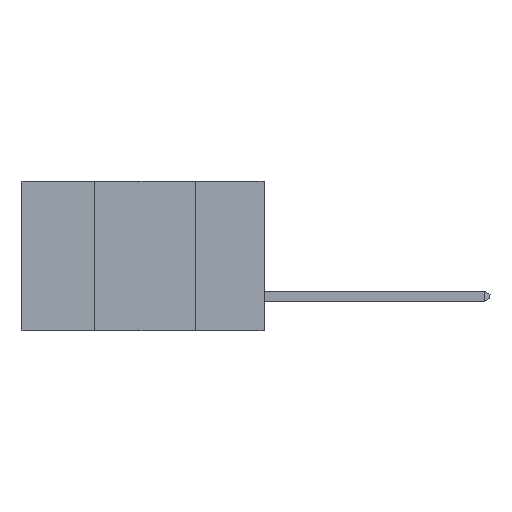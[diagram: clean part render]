
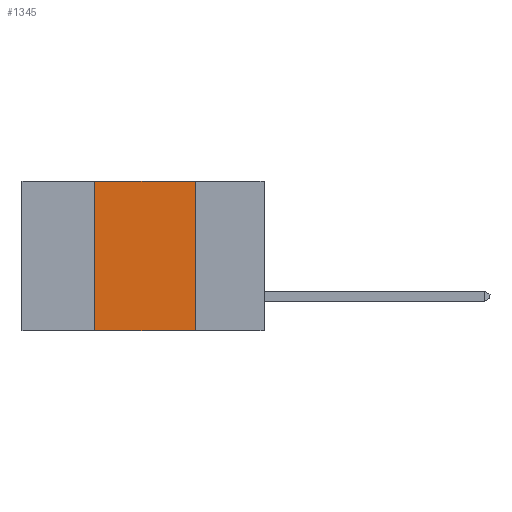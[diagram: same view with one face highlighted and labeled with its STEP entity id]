
A CAD part, left-side view. The second image highlights one B-rep face of the part: STEP entity #1345.
In plain terms, the highlighted planar face has unit normal (-1, 0, 0).
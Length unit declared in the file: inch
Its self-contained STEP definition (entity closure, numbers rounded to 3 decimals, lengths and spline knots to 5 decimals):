
#128 = ORIENTED_EDGE ( 'NONE', *, *, #4056, .F. ) ;
#485 = EDGE_LOOP ( 'NONE', ( #1250, #128, #4569, #4271 ) ) ;
#500 = FACE_OUTER_BOUND ( 'NONE', #485, .T. ) ;
#952 = VECTOR ( 'NONE', #2828, 39.37008 ) ;
#1250 = ORIENTED_EDGE ( 'NONE', *, *, #1467, .F. ) ;
#1345 = ADVANCED_FACE ( 'NONE', ( #500 ), #5848, .F. ) ;
#1467 = EDGE_CURVE ( 'NONE', #7195, #2257, #3951, .T. ) ;
#1791 = DIRECTION ( 'NONE',  ( 0., 0., -1. ) ) ;
#1804 = VECTOR ( 'NONE', #7386, 39.37008 ) ;
#1871 = CARTESIAN_POINT ( 'NONE',  ( 0., 0.6, 0. ) ) ;
#1901 = CARTESIAN_POINT ( 'NONE',  ( 0., 0.6, -0.37 ) ) ;
#1982 = CARTESIAN_POINT ( 'NONE',  ( 0., 0.42, 0. ) ) ;
#2257 = VERTEX_POINT ( 'NONE', #8460 ) ;
#2698 = CARTESIAN_POINT ( 'NONE',  ( 0., 0.17, -0.37 ) ) ;
#2828 = DIRECTION ( 'NONE',  ( 0., 0., -1. ) ) ;
#3040 = DIRECTION ( 'NONE',  ( 0., -1., 0. ) ) ;
#3544 = LINE ( 'NONE', #3629, #1804 ) ;
#3629 = CARTESIAN_POINT ( 'NONE',  ( 0., 0.42, -0.37 ) ) ;
#3779 = VERTEX_POINT ( 'NONE', #1982 ) ;
#3916 = CARTESIAN_POINT ( 'NONE',  ( 0., 0.17, 0. ) ) ;
#3951 = LINE ( 'NONE', #2698, #952 ) ;
#4056 = EDGE_CURVE ( 'NONE', #3779, #7195, #7327, .T. ) ;
#4271 = ORIENTED_EDGE ( 'NONE', *, *, #4809, .T. ) ;
#4569 = ORIENTED_EDGE ( 'NONE', *, *, #5595, .F. ) ;
#4743 = VERTEX_POINT ( 'NONE', #5188 ) ;
#4809 = EDGE_CURVE ( 'NONE', #4743, #2257, #5022, .T. ) ;
#5022 = LINE ( 'NONE', #1901, #8263 ) ;
#5188 = CARTESIAN_POINT ( 'NONE',  ( 0., 0.42, -0.37 ) ) ;
#5595 = EDGE_CURVE ( 'NONE', #4743, #3779, #3544, .T. ) ;
#5820 = DIRECTION ( 'NONE',  ( 0., -1., 0. ) ) ;
#5848 = PLANE ( 'NONE',  #6576 ) ;
#5886 = DIRECTION ( 'NONE',  ( 1., 0., 0. ) ) ;
#6112 = CARTESIAN_POINT ( 'NONE',  ( 0., 0.6, 0. ) ) ;
#6576 = AXIS2_PLACEMENT_3D ( 'NONE', #1871, #5886, #1791 ) ;
#7158 = VECTOR ( 'NONE', #5820, 39.37008 ) ;
#7195 = VERTEX_POINT ( 'NONE', #3916 ) ;
#7327 = LINE ( 'NONE', #6112, #7158 ) ;
#7386 = DIRECTION ( 'NONE',  ( 0., 0., 1. ) ) ;
#8263 = VECTOR ( 'NONE', #3040, 39.37008 ) ;
#8460 = CARTESIAN_POINT ( 'NONE',  ( 0., 0.17, -0.37 ) ) ;
